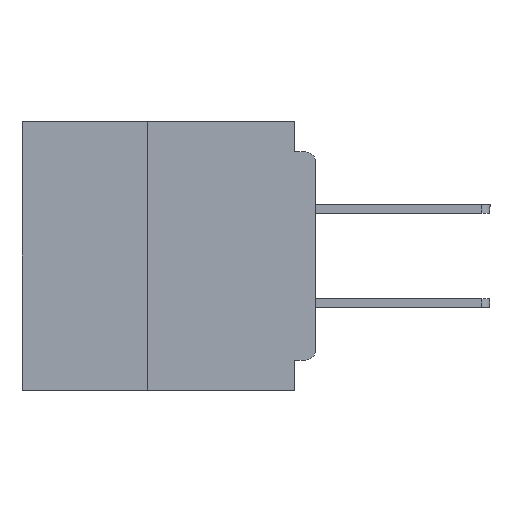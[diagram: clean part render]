
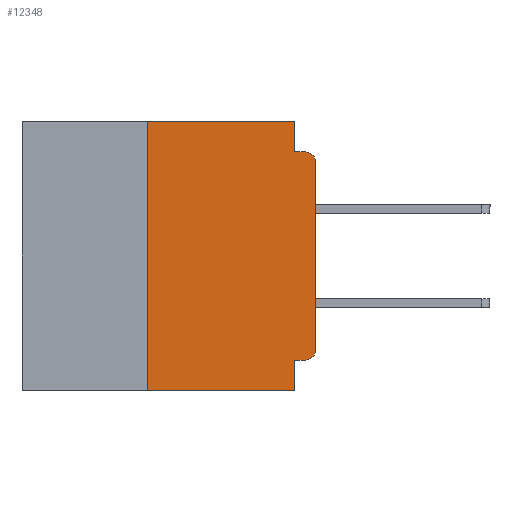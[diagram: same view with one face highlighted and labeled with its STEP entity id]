
A CAD part, left-side view. The second image highlights one B-rep face of the part: STEP entity #12348.
In plain terms, the highlighted planar face has unit normal (-1, 0, 0).
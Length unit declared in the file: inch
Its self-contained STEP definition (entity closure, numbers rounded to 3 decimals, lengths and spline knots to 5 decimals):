
#16 = ORIENTED_EDGE ( 'NONE', *, *, #38736, .F. ) ;
#41 = VERTEX_POINT ( 'NONE', #36478 ) ;
#360 = AXIS2_PLACEMENT_3D ( 'NONE', #9889, #31582, #13031 ) ;
#603 = CARTESIAN_POINT ( 'NONE',  ( 0., 0.437, 0. ) ) ;
#713 = VERTEX_POINT ( 'NONE', #5876 ) ;
#766 = ORIENTED_EDGE ( 'NONE', *, *, #4953, .F. ) ;
#2510 = VERTEX_POINT ( 'NONE', #22640 ) ;
#2529 = CARTESIAN_POINT ( 'NONE',  ( 0., 0., -0.045 ) ) ;
#2907 = ORIENTED_EDGE ( 'NONE', *, *, #12379, .T. ) ;
#3991 = ORIENTED_EDGE ( 'NONE', *, *, #22812, .F. ) ;
#4953 = EDGE_CURVE ( 'NONE', #713, #5889, #19441, .T. ) ;
#5384 = CARTESIAN_POINT ( 'NONE',  ( 0., 0., -0.355 ) ) ;
#5876 = CARTESIAN_POINT ( 'NONE',  ( 0., 0.25, -0.4 ) ) ;
#5889 = VERTEX_POINT ( 'NONE', #24142 ) ;
#6230 = DIRECTION ( 'NONE',  ( 0., 0., 1. ) ) ;
#6313 = EDGE_LOOP ( 'NONE', ( #8824, #17098, #10803, #27254, #16, #766, #2907, #3991, #6693, #7232 ) ) ;
#6693 = ORIENTED_EDGE ( 'NONE', *, *, #35475, .F. ) ;
#7232 = ORIENTED_EDGE ( 'NONE', *, *, #21843, .T. ) ;
#7335 = LINE ( 'NONE', #16681, #23855 ) ;
#7888 = LINE ( 'NONE', #22552, #23426 ) ;
#8824 = ORIENTED_EDGE ( 'NONE', *, *, #12879, .T. ) ;
#9889 = CARTESIAN_POINT ( 'NONE',  ( 0., 0.015, -0.34 ) ) ;
#10059 = DIRECTION ( 'NONE',  ( 1., 0., 0. ) ) ;
#10803 = ORIENTED_EDGE ( 'NONE', *, *, #36784, .F. ) ;
#11097 = CARTESIAN_POINT ( 'NONE',  ( 0., 0.015, -0.045 ) ) ;
#11264 = CARTESIAN_POINT ( 'NONE',  ( 0., 0., -0.06 ) ) ;
#11473 = CARTESIAN_POINT ( 'NONE',  ( 0., 0.031, -0.4 ) ) ;
#11854 = VERTEX_POINT ( 'NONE', #13913 ) ;
#11964 = DIRECTION ( 'NONE',  ( 0., -1., 0. ) ) ;
#12167 = VECTOR ( 'NONE', #29684, 39.37008 ) ;
#12348 = ADVANCED_FACE ( 'NONE', ( #25360 ), #34606, .F. ) ;
#12379 = EDGE_CURVE ( 'NONE', #713, #11854, #7888, .T. ) ;
#12497 = CARTESIAN_POINT ( 'NONE',  ( 0., 0., 0. ) ) ;
#12879 = EDGE_CURVE ( 'NONE', #26444, #33016, #30652, .T. ) ;
#13031 = DIRECTION ( 'NONE',  ( 0., 0., -1. ) ) ;
#13216 = VECTOR ( 'NONE', #6230, 39.37008 ) ;
#13913 = CARTESIAN_POINT ( 'NONE',  ( 0., 0.031, -0.4 ) ) ;
#14782 = EDGE_CURVE ( 'NONE', #20147, #41, #7335, .T. ) ;
#15209 = DIRECTION ( 'NONE',  ( -1., 0., 0. ) ) ;
#15351 = LINE ( 'NONE', #11473, #37965 ) ;
#16681 = CARTESIAN_POINT ( 'NONE',  ( 0., 0.031, 0. ) ) ;
#17098 = ORIENTED_EDGE ( 'NONE', *, *, #26871, .T. ) ;
#19092 = VECTOR ( 'NONE', #11964, 39.37008 ) ;
#19337 = CIRCLE ( 'NONE', #360, 0.015 ) ;
#19441 = LINE ( 'NONE', #29676, #12167 ) ;
#19824 = DIRECTION ( 'NONE',  ( 0., 0., -1. ) ) ;
#20147 = VERTEX_POINT ( 'NONE', #24342 ) ;
#21843 = EDGE_CURVE ( 'NONE', #33393, #26444, #19337, .T. ) ;
#22552 = CARTESIAN_POINT ( 'NONE',  ( 0., 0.437, -0.4 ) ) ;
#22640 = CARTESIAN_POINT ( 'NONE',  ( 0., 0.031, -0.355 ) ) ;
#22812 = EDGE_CURVE ( 'NONE', #2510, #11854, #15351, .T. ) ;
#22916 = CARTESIAN_POINT ( 'NONE',  ( 0., 0.437, 0. ) ) ;
#23426 = VECTOR ( 'NONE', #28747, 39.37008 ) ;
#23434 = AXIS2_PLACEMENT_3D ( 'NONE', #33667, #15209, #36725 ) ;
#23855 = VECTOR ( 'NONE', #19824, 39.37008 ) ;
#24142 = CARTESIAN_POINT ( 'NONE',  ( 0., 0.25, 0. ) ) ;
#24342 = CARTESIAN_POINT ( 'NONE',  ( 0., 0.031, 0. ) ) ;
#25360 = FACE_OUTER_BOUND ( 'NONE', #6313, .T. ) ;
#26444 = VERTEX_POINT ( 'NONE', #28238 ) ;
#26871 = EDGE_CURVE ( 'NONE', #33016, #29949, #35536, .T. ) ;
#27254 = ORIENTED_EDGE ( 'NONE', *, *, #14782, .F. ) ;
#27296 = LINE ( 'NONE', #2529, #19092 ) ;
#28238 = CARTESIAN_POINT ( 'NONE',  ( 0., 0., -0.34 ) ) ;
#28677 = CARTESIAN_POINT ( 'NONE',  ( 0., 0.015, -0.355 ) ) ;
#28747 = DIRECTION ( 'NONE',  ( 0., -1., 0. ) ) ;
#29055 = VECTOR ( 'NONE', #32216, 39.37008 ) ;
#29676 = CARTESIAN_POINT ( 'NONE',  ( 0., 0.25, -0.4 ) ) ;
#29684 = DIRECTION ( 'NONE',  ( 0., 0., 1. ) ) ;
#29949 = VERTEX_POINT ( 'NONE', #11097 ) ;
#30016 = DIRECTION ( 'NONE',  ( 0., 0., -1. ) ) ;
#30199 = DIRECTION ( 'NONE',  ( 0., 1., 0. ) ) ;
#30652 = LINE ( 'NONE', #12497, #13216 ) ;
#31014 = LINE ( 'NONE', #22916, #29055 ) ;
#31582 = DIRECTION ( 'NONE',  ( -1., 0., 0. ) ) ;
#31732 = DIRECTION ( 'NONE',  ( 0., 0., -1. ) ) ;
#32216 = DIRECTION ( 'NONE',  ( 0., -1., 0. ) ) ;
#33016 = VERTEX_POINT ( 'NONE', #11264 ) ;
#33393 = VERTEX_POINT ( 'NONE', #28677 ) ;
#33632 = VECTOR ( 'NONE', #30199, 39.37008 ) ;
#33667 = CARTESIAN_POINT ( 'NONE',  ( 0., 0.015, -0.06 ) ) ;
#34593 = LINE ( 'NONE', #5384, #33632 ) ;
#34606 = PLANE ( 'NONE',  #35636 ) ;
#35475 = EDGE_CURVE ( 'NONE', #33393, #2510, #34593, .T. ) ;
#35536 = CIRCLE ( 'NONE', #23434, 0.015 ) ;
#35636 = AXIS2_PLACEMENT_3D ( 'NONE', #603, #10059, #31732 ) ;
#36478 = CARTESIAN_POINT ( 'NONE',  ( 0., 0.031, -0.045 ) ) ;
#36725 = DIRECTION ( 'NONE',  ( 0., 0., -1. ) ) ;
#36784 = EDGE_CURVE ( 'NONE', #41, #29949, #27296, .T. ) ;
#37965 = VECTOR ( 'NONE', #30016, 39.37008 ) ;
#38736 = EDGE_CURVE ( 'NONE', #5889, #20147, #31014, .T. ) ;
